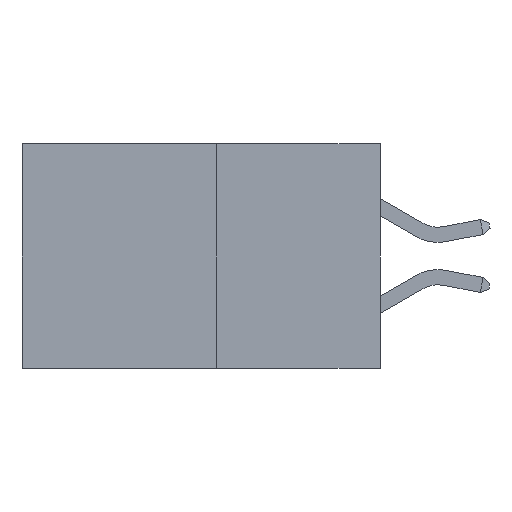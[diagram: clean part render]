
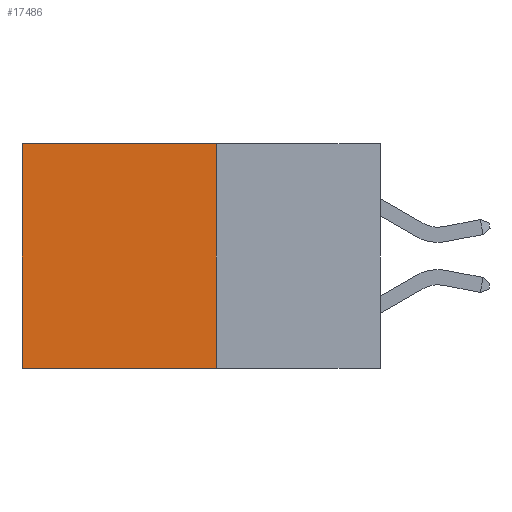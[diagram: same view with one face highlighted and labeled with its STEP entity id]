
A CAD part, left-side view. The second image highlights one B-rep face of the part: STEP entity #17486.
In plain terms, the highlighted planar face has unit normal (-1, 0, 0).
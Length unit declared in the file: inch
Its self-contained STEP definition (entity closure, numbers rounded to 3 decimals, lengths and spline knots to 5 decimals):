
#288 = LINE ( 'NONE', #6398, #14407 ) ;
#1087 = VECTOR ( 'NONE', #14861, 39.37008 ) ;
#1553 = VERTEX_POINT ( 'NONE', #10395 ) ;
#1893 = EDGE_LOOP ( 'NONE', ( #10497, #2149, #22902, #17630 ) ) ;
#1919 = EDGE_CURVE ( 'NONE', #14591, #4474, #14798, .T. ) ;
#2149 = ORIENTED_EDGE ( 'NONE', *, *, #4816, .F. ) ;
#2390 = PLANE ( 'NONE',  #8510 ) ;
#2734 = VERTEX_POINT ( 'NONE', #7896 ) ;
#3823 = CARTESIAN_POINT ( 'NONE',  ( 0.277, 0.27, -0.37 ) ) ;
#4041 = CARTESIAN_POINT ( 'NONE',  ( 0.277, 0.59, -0.37 ) ) ;
#4474 = VERTEX_POINT ( 'NONE', #4041 ) ;
#4816 = EDGE_CURVE ( 'NONE', #2734, #4474, #22469, .T. ) ;
#5468 = CARTESIAN_POINT ( 'NONE',  ( 0.277, 0.59, 0. ) ) ;
#5810 = FACE_OUTER_BOUND ( 'NONE', #1893, .T. ) ;
#6170 = CARTESIAN_POINT ( 'NONE',  ( 0.277, 0.27, -0.37 ) ) ;
#6398 = CARTESIAN_POINT ( 'NONE',  ( 0.277, 0.27, 0. ) ) ;
#7896 = CARTESIAN_POINT ( 'NONE',  ( 0.277, 0.27, -0.37 ) ) ;
#8050 = DIRECTION ( 'NONE',  ( 0., 0., -1. ) ) ;
#8276 = DIRECTION ( 'NONE',  ( 0., 1., 0. ) ) ;
#8510 = AXIS2_PLACEMENT_3D ( 'NONE', #6170, #18861, #8050 ) ;
#10395 = CARTESIAN_POINT ( 'NONE',  ( 0.277, 0.27, 0. ) ) ;
#10497 = ORIENTED_EDGE ( 'NONE', *, *, #1919, .T. ) ;
#11237 = EDGE_CURVE ( 'NONE', #1553, #14591, #288, .T. ) ;
#11523 = LINE ( 'NONE', #3823, #1087 ) ;
#12743 = EDGE_CURVE ( 'NONE', #1553, #2734, #11523, .T. ) ;
#14407 = VECTOR ( 'NONE', #8276, 39.37008 ) ;
#14591 = VERTEX_POINT ( 'NONE', #5468 ) ;
#14798 = LINE ( 'NONE', #16545, #19589 ) ;
#14861 = DIRECTION ( 'NONE',  ( 0., 0., -1. ) ) ;
#16545 = CARTESIAN_POINT ( 'NONE',  ( 0.277, 0.59, -0.37 ) ) ;
#17486 = ADVANCED_FACE ( 'NONE', ( #5810 ), #2390, .F. ) ;
#17630 = ORIENTED_EDGE ( 'NONE', *, *, #11237, .T. ) ;
#18618 = CARTESIAN_POINT ( 'NONE',  ( 0.277, 0.27, -0.37 ) ) ;
#18861 = DIRECTION ( 'NONE',  ( 1., 0., 0. ) ) ;
#19256 = DIRECTION ( 'NONE',  ( 0., 1., 0. ) ) ;
#19589 = VECTOR ( 'NONE', #20778, 39.37008 ) ;
#20494 = VECTOR ( 'NONE', #19256, 39.37008 ) ;
#20778 = DIRECTION ( 'NONE',  ( 0., 0., -1. ) ) ;
#22469 = LINE ( 'NONE', #18618, #20494 ) ;
#22902 = ORIENTED_EDGE ( 'NONE', *, *, #12743, .F. ) ;
